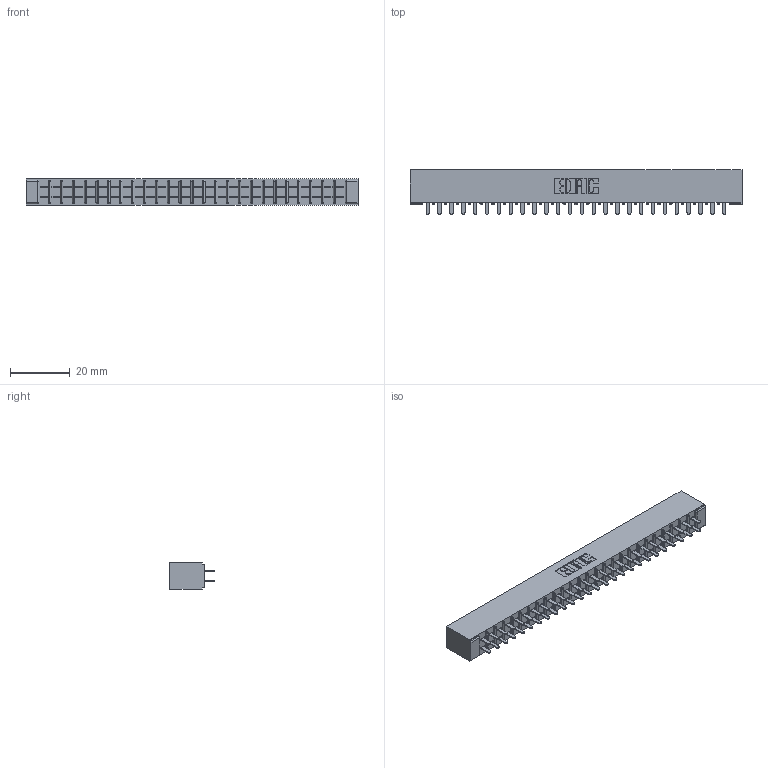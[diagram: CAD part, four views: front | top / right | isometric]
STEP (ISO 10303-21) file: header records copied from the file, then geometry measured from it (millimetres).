
FILE_DESCRIPTION (( 'STEP AP203' ), '1' );
FILE_NAME ('355-052-521-501.STEP', '2019-09-11T16:28:07', ( '' ), ( '' ), 'SwSTEP 2.0', 'SolidWorks 2016', '' );
FILE_SCHEMA (( 'CONFIG_CONTROL_DESIGN' ));
Length unit declared in the file: inch
Products named in the file (3): 355-052-521-501; 305 Part_No Mounting; 305-290-001_521
Assembly tree (53 placements, depth 2):
  355-052-521-501
    305 Part_No Mounting
    305-290-001_521  x52
Bounding box: 110.9 x 14.86 x 8.71 mm (x, y, z)
Volume: 6729.9 mm3; surface area: 14093.5 mm2
Topology: 53 solids, 53 shells, 2500 faces, 7130 edges, 4612 vertices
Faces by surface type: plane 1468, cylinder 928, sphere 104
Entity records: 29701 total; most frequent: CARTESIAN_POINT 4912, ORIENTED_EDGE 4872, DIRECTION 4762, EDGE_CURVE 2436, VECTOR 1958, LINE 1958, VERTEX_POINT 1552, AXIS2_PLACEMENT_3D 1402
